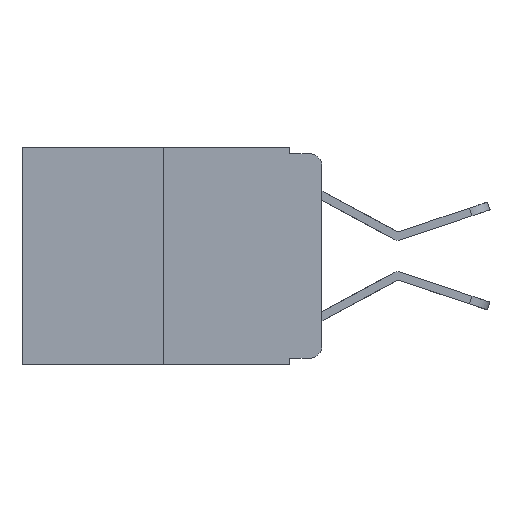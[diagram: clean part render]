
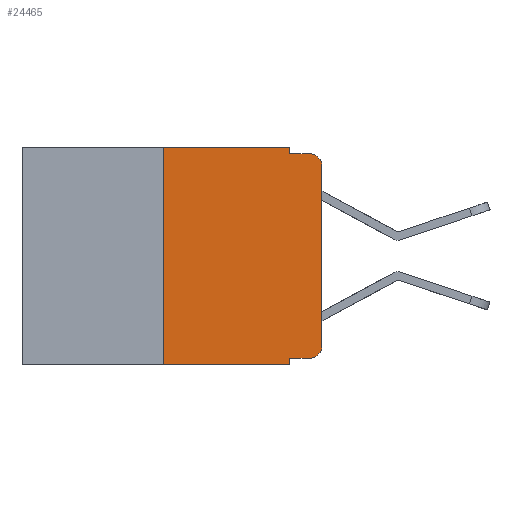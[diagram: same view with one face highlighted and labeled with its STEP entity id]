
A CAD part, left-side view. The second image highlights one B-rep face of the part: STEP entity #24465.
In plain terms, the highlighted planar face has unit normal (-1, 0, 0).
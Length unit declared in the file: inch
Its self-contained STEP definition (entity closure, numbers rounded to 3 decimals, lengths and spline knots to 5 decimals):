
#56 = CARTESIAN_POINT ( 'NONE',  ( 0., 0.02, -0.333 ) ) ;
#532 = DIRECTION ( 'NONE',  ( 0., -1., 0. ) ) ;
#747 = LINE ( 'NONE', #13085, #16504 ) ;
#1092 = VECTOR ( 'NONE', #1962, 39.37008 ) ;
#1521 = LINE ( 'NONE', #10808, #11103 ) ;
#1962 = DIRECTION ( 'NONE',  ( 0., 0., 1. ) ) ;
#2128 = VECTOR ( 'NONE', #532, 39.37008 ) ;
#2541 = VERTEX_POINT ( 'NONE', #15210 ) ;
#2580 = CARTESIAN_POINT ( 'NONE',  ( 0., 0., -0.313 ) ) ;
#2682 = EDGE_CURVE ( 'NONE', #13639, #19161, #16164, .T. ) ;
#2748 = ORIENTED_EDGE ( 'NONE', *, *, #5403, .F. ) ;
#3173 = ORIENTED_EDGE ( 'NONE', *, *, #7966, .T. ) ;
#3436 = DIRECTION ( 'NONE',  ( -1., 0., 0. ) ) ;
#3564 = EDGE_LOOP ( 'NONE', ( #4220, #5506, #9282, #10227, #16300, #2748, #6460, #10879, #10212, #3173 ) ) ;
#3774 = AXIS2_PLACEMENT_3D ( 'NONE', #9186, #22192, #11060 ) ;
#3881 = FACE_OUTER_BOUND ( 'NONE', #3564, .T. ) ;
#4220 = ORIENTED_EDGE ( 'NONE', *, *, #22929, .T. ) ;
#5403 = EDGE_CURVE ( 'NONE', #13639, #5936, #16025, .T. ) ;
#5506 = ORIENTED_EDGE ( 'NONE', *, *, #19211, .T. ) ;
#5540 = DIRECTION ( 'NONE',  ( 0., -1., 0. ) ) ;
#5650 = AXIS2_PLACEMENT_3D ( 'NONE', #14658, #3436, #16584 ) ;
#5919 = AXIS2_PLACEMENT_3D ( 'NONE', #20071, #10800, #23790 ) ;
#5936 = VERTEX_POINT ( 'NONE', #19890 ) ;
#6460 = ORIENTED_EDGE ( 'NONE', *, *, #2682, .T. ) ;
#6543 = CARTESIAN_POINT ( 'NONE',  ( 0., 0.25, -0.343 ) ) ;
#7452 = VERTEX_POINT ( 'NONE', #13262 ) ;
#7966 = EDGE_CURVE ( 'NONE', #16275, #18928, #24265, .T. ) ;
#8200 = DIRECTION ( 'NONE',  ( 0., 0., -1. ) ) ;
#9186 = CARTESIAN_POINT ( 'NONE',  ( 0., 0.02, -0.313 ) ) ;
#9282 = ORIENTED_EDGE ( 'NONE', *, *, #10483, .F. ) ;
#10179 = LINE ( 'NONE', #18742, #24407 ) ;
#10212 = ORIENTED_EDGE ( 'NONE', *, *, #20910, .T. ) ;
#10227 = ORIENTED_EDGE ( 'NONE', *, *, #17966, .F. ) ;
#10314 = VERTEX_POINT ( 'NONE', #15260 ) ;
#10483 = EDGE_CURVE ( 'NONE', #10314, #20830, #17768, .T. ) ;
#10800 = DIRECTION ( 'NONE',  ( 1., 0., 0. ) ) ;
#10808 = CARTESIAN_POINT ( 'NONE',  ( 0., 0.051, -0.333 ) ) ;
#10879 = ORIENTED_EDGE ( 'NONE', *, *, #11718, .F. ) ;
#11060 = DIRECTION ( 'NONE',  ( 0., 0., -1. ) ) ;
#11103 = VECTOR ( 'NONE', #12664, 39.37008 ) ;
#11718 = EDGE_CURVE ( 'NONE', #17470, #19161, #14455, .T. ) ;
#12221 = DIRECTION ( 'NONE',  ( 0., -1., 0. ) ) ;
#12664 = DIRECTION ( 'NONE',  ( 0., -1., 0. ) ) ;
#13085 = CARTESIAN_POINT ( 'NONE',  ( 0., 0.473, 0. ) ) ;
#13262 = CARTESIAN_POINT ( 'NONE',  ( 0., 0., -0.03 ) ) ;
#13639 = VERTEX_POINT ( 'NONE', #6543 ) ;
#13942 = EDGE_CURVE ( 'NONE', #5936, #2541, #747, .T. ) ;
#14455 = LINE ( 'NONE', #23090, #18284 ) ;
#14658 = CARTESIAN_POINT ( 'NONE',  ( 0., 0.02, -0.03 ) ) ;
#14906 = CARTESIAN_POINT ( 'NONE',  ( 0., 0.473, -0.343 ) ) ;
#14935 = CIRCLE ( 'NONE', #5650, 0.02 ) ;
#15210 = CARTESIAN_POINT ( 'NONE',  ( 0., 0.051, 0. ) ) ;
#15260 = CARTESIAN_POINT ( 'NONE',  ( 0., 0.051, -0.01 ) ) ;
#15628 = CARTESIAN_POINT ( 'NONE',  ( 0., 0.25, 0. ) ) ;
#15669 = CARTESIAN_POINT ( 'NONE',  ( 0., 0.051, -0.01 ) ) ;
#16025 = LINE ( 'NONE', #15628, #20392 ) ;
#16164 = LINE ( 'NONE', #14906, #20530 ) ;
#16233 = LINE ( 'NONE', #24443, #1092 ) ;
#16275 = VERTEX_POINT ( 'NONE', #56 ) ;
#16300 = ORIENTED_EDGE ( 'NONE', *, *, #13942, .F. ) ;
#16504 = VECTOR ( 'NONE', #5540, 39.37008 ) ;
#16584 = DIRECTION ( 'NONE',  ( 0., 0., -1. ) ) ;
#16760 = DIRECTION ( 'NONE',  ( 0., 0., 1. ) ) ;
#17470 = VERTEX_POINT ( 'NONE', #22892 ) ;
#17768 = LINE ( 'NONE', #15669, #2128 ) ;
#17966 = EDGE_CURVE ( 'NONE', #2541, #10314, #10179, .T. ) ;
#18211 = PLANE ( 'NONE',  #5919 ) ;
#18284 = VECTOR ( 'NONE', #8200, 39.37008 ) ;
#18742 = CARTESIAN_POINT ( 'NONE',  ( 0., 0.051, 0. ) ) ;
#18928 = VERTEX_POINT ( 'NONE', #2580 ) ;
#19161 = VERTEX_POINT ( 'NONE', #21933 ) ;
#19211 = EDGE_CURVE ( 'NONE', #7452, #20830, #14935, .T. ) ;
#19839 = CARTESIAN_POINT ( 'NONE',  ( 0., 0.02, -0.01 ) ) ;
#19890 = CARTESIAN_POINT ( 'NONE',  ( 0., 0.25, 0. ) ) ;
#20071 = CARTESIAN_POINT ( 'NONE',  ( 0., 0.473, 0. ) ) ;
#20392 = VECTOR ( 'NONE', #16760, 39.37008 ) ;
#20530 = VECTOR ( 'NONE', #12221, 39.37008 ) ;
#20604 = DIRECTION ( 'NONE',  ( 0., 0., -1. ) ) ;
#20830 = VERTEX_POINT ( 'NONE', #19839 ) ;
#20910 = EDGE_CURVE ( 'NONE', #17470, #16275, #1521, .T. ) ;
#21933 = CARTESIAN_POINT ( 'NONE',  ( 0., 0.051, -0.343 ) ) ;
#22192 = DIRECTION ( 'NONE',  ( -1., 0., 0. ) ) ;
#22892 = CARTESIAN_POINT ( 'NONE',  ( 0., 0.051, -0.333 ) ) ;
#22929 = EDGE_CURVE ( 'NONE', #18928, #7452, #16233, .T. ) ;
#23090 = CARTESIAN_POINT ( 'NONE',  ( 0., 0.051, 0. ) ) ;
#23790 = DIRECTION ( 'NONE',  ( 0., 0., -1. ) ) ;
#24265 = CIRCLE ( 'NONE', #3774, 0.02 ) ;
#24407 = VECTOR ( 'NONE', #20604, 39.37008 ) ;
#24443 = CARTESIAN_POINT ( 'NONE',  ( 0., 0., 0. ) ) ;
#24465 = ADVANCED_FACE ( 'NONE', ( #3881 ), #18211, .F. ) ;
